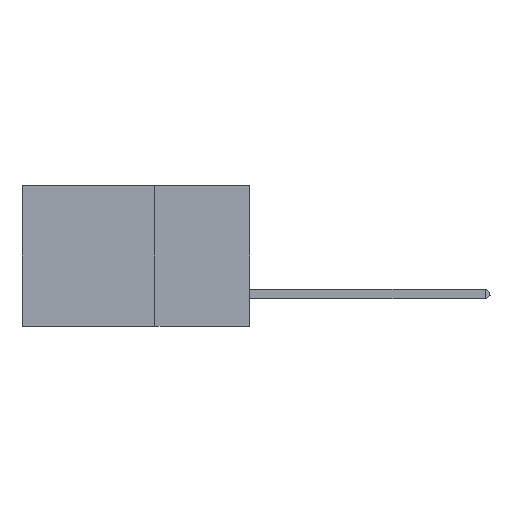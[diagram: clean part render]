
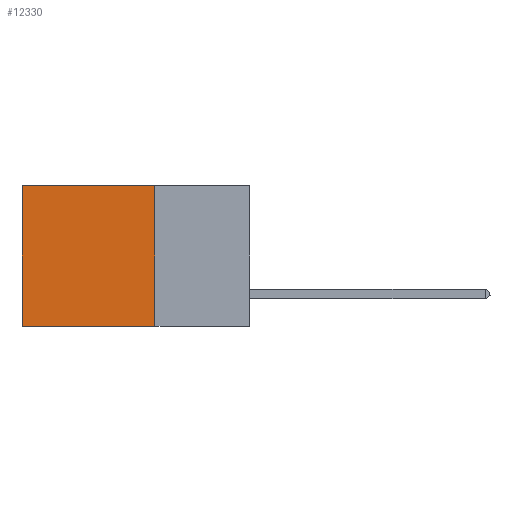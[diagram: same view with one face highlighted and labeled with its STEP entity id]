
A CAD part, left-side view. The second image highlights one B-rep face of the part: STEP entity #12330.
In plain terms, the highlighted planar face has unit normal (-1, 0, 0).
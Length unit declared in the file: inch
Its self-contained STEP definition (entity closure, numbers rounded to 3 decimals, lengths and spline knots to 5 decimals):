
#7 = EDGE_CURVE ( 'NONE', #5607, #4164, #8048, .T. ) ;
#96 = VECTOR ( 'NONE', #8817, 39.37008 ) ;
#150 = ORIENTED_EDGE ( 'NONE', *, *, #15651, .F. ) ;
#421 = CARTESIAN_POINT ( 'NONE',  ( 0.2875, 0.25, 0. ) ) ;
#525 = EDGE_CURVE ( 'NONE', #16813, #8864, #9723, .T. ) ;
#1964 = VECTOR ( 'NONE', #10142, 39.37008 ) ;
#1975 = VECTOR ( 'NONE', #4844, 39.37008 ) ;
#2215 = CARTESIAN_POINT ( 'NONE',  ( 0.2875, 0.25, 0. ) ) ;
#2456 = VECTOR ( 'NONE', #13966, 39.37008 ) ;
#2527 = ORIENTED_EDGE ( 'NONE', *, *, #525, .T. ) ;
#3457 = CARTESIAN_POINT ( 'NONE',  ( 0.2875, 0.6, 0. ) ) ;
#4164 = VERTEX_POINT ( 'NONE', #4557 ) ;
#4557 = CARTESIAN_POINT ( 'NONE',  ( 0.2875, 0.6, -0.37 ) ) ;
#4740 = ORIENTED_EDGE ( 'NONE', *, *, #7, .F. ) ;
#4844 = DIRECTION ( 'NONE',  ( 0., 0., -1. ) ) ;
#5607 = VERTEX_POINT ( 'NONE', #12738 ) ;
#5832 = DIRECTION ( 'NONE',  ( 1., 0., 0. ) ) ;
#6898 = PLANE ( 'NONE',  #11795 ) ;
#8048 = LINE ( 'NONE', #10027, #1964 ) ;
#8055 = EDGE_CURVE ( 'NONE', #8864, #4164, #9241, .T. ) ;
#8817 = DIRECTION ( 'NONE',  ( 0., 0., -1. ) ) ;
#8864 = VERTEX_POINT ( 'NONE', #3457 ) ;
#9241 = LINE ( 'NONE', #9876, #96 ) ;
#9716 = DIRECTION ( 'NONE',  ( 0., 0., -1. ) ) ;
#9723 = LINE ( 'NONE', #2215, #2456 ) ;
#9876 = CARTESIAN_POINT ( 'NONE',  ( 0.2875, 0.6, 0. ) ) ;
#10027 = CARTESIAN_POINT ( 'NONE',  ( 0.2875, 0.25, -0.37 ) ) ;
#10142 = DIRECTION ( 'NONE',  ( 0., 1., 0. ) ) ;
#10499 = FACE_OUTER_BOUND ( 'NONE', #15378, .T. ) ;
#11047 = LINE ( 'NONE', #16584, #1975 ) ;
#11795 = AXIS2_PLACEMENT_3D ( 'NONE', #421, #5832, #9716 ) ;
#12330 = ADVANCED_FACE ( 'NONE', ( #10499 ), #6898, .F. ) ;
#12593 = ORIENTED_EDGE ( 'NONE', *, *, #8055, .T. ) ;
#12738 = CARTESIAN_POINT ( 'NONE',  ( 0.2875, 0.25, -0.37 ) ) ;
#13966 = DIRECTION ( 'NONE',  ( 0., 1., 0. ) ) ;
#15378 = EDGE_LOOP ( 'NONE', ( #12593, #4740, #150, #2527 ) ) ;
#15651 = EDGE_CURVE ( 'NONE', #16813, #5607, #11047, .T. ) ;
#16584 = CARTESIAN_POINT ( 'NONE',  ( 0.2875, 0.25, 0. ) ) ;
#16599 = CARTESIAN_POINT ( 'NONE',  ( 0.2875, 0.25, 0. ) ) ;
#16813 = VERTEX_POINT ( 'NONE', #16599 ) ;
